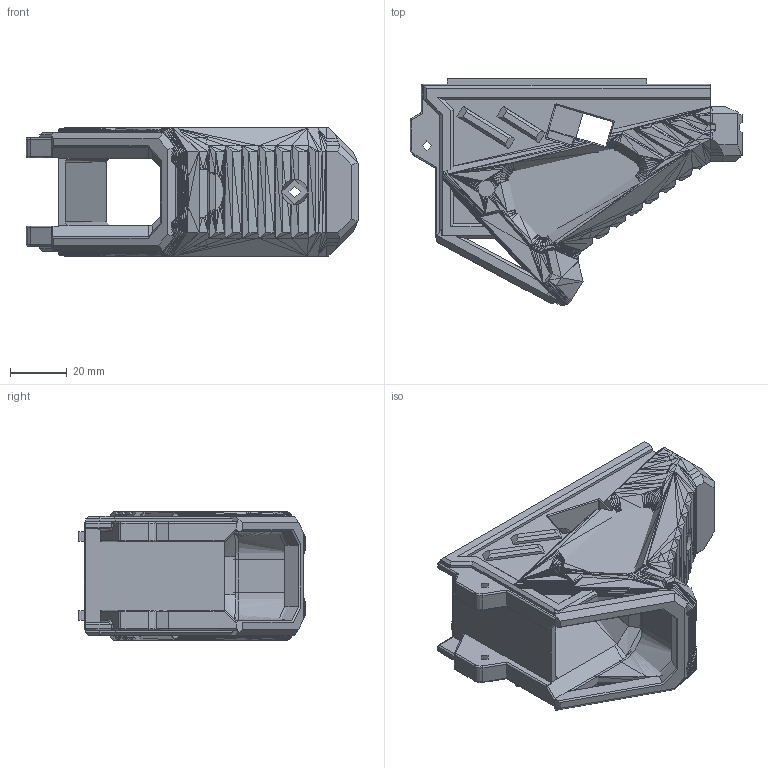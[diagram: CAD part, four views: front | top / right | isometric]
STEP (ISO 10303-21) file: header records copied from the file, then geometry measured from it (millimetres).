
FILE_DESCRIPTION(/* description */ (''),/* implementation_level */ '2;1');
FILE_NAME(/* name */ 'MOD9_magwell_GOAT V3 v13.step',/* time_stamp */ '2020-09-02T19:53:15-05:00',/* author */ (''),/* organization */ (''),/* preprocessor_version */ 'ST-DEVELOPER v18.1',/* originating_system */ 'Autodesk Translation Framework v9.3.0.1241',/* authorisation */ '');
FILE_SCHEMA (('AUTOMOTIVE_DESIGN { 1 0 10303 214 3 1 1 }'));
Products named in the file (1): MOD9_magwell_GOAT V3
Bounding box: 116.51 x 79.5 x 44.94 mm (x, y, z)
Volume: 170747.5 mm3
Topology: 2 solids, 9 shells, 2285 faces, 4718 edges, 2446 vertices
Faces by surface type: plane 2107, cylinder 91, bspline 66, torus 13, sphere 6, cone 2
Full cylindrical faces by diameter (mm): 1.5 x2, 3.4 x2, 4 x2, 9 x1
Entity records: 58856 total; most frequent: CARTESIAN_POINT 12252, ORIENTED_EDGE 9442, DIRECTION 9269, EDGE_CURVE 4721, LINE 4279, VECTOR 4279, AXIS2_PLACEMENT_3D 2495, VERTEX_POINT 2446
